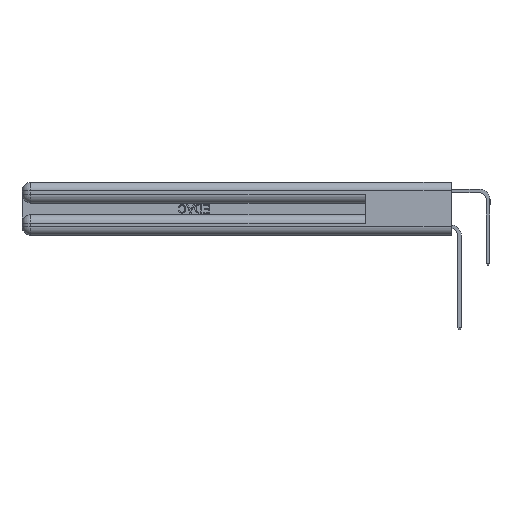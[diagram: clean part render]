
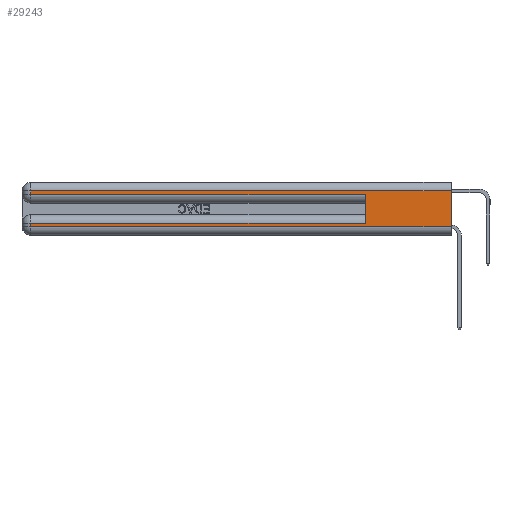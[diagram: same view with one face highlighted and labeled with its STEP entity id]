
A CAD part, left-side view. The second image highlights one B-rep face of the part: STEP entity #29243.
In plain terms, the highlighted planar face has unit normal (-1, 0, 0).
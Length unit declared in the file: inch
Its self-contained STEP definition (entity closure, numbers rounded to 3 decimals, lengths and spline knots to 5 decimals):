
#84 = LINE ( 'NONE', #25283, #3371 ) ;
#491 = LINE ( 'NONE', #1988, #9873 ) ;
#773 = EDGE_CURVE ( 'NONE', #15879, #17200, #33847, .T. ) ;
#850 = CARTESIAN_POINT ( 'NONE',  ( 0., 2.94, 0.37 ) ) ;
#945 = EDGE_LOOP ( 'NONE', ( #5033, #32286, #2455, #17928, #13160, #16162, #26212, #3657 ) ) ;
#1550 = CARTESIAN_POINT ( 'NONE',  ( 0., 2.94, 0.085 ) ) ;
#1559 = DIRECTION ( 'NONE',  ( 1., 0., 0. ) ) ;
#1988 = CARTESIAN_POINT ( 'NONE',  ( 0., 0., 0.085 ) ) ;
#2306 = CARTESIAN_POINT ( 'NONE',  ( 0., 2.94, 0.285 ) ) ;
#2379 = CARTESIAN_POINT ( 'NONE',  ( 0., 0.6, 0.085 ) ) ;
#2455 = ORIENTED_EDGE ( 'NONE', *, *, #14987, .T. ) ;
#3231 = LINE ( 'NONE', #850, #30244 ) ;
#3371 = VECTOR ( 'NONE', #14775, 39.37008 ) ;
#3577 = EDGE_CURVE ( 'NONE', #5012, #21733, #84, .T. ) ;
#3657 = ORIENTED_EDGE ( 'NONE', *, *, #11241, .T. ) ;
#4285 = CARTESIAN_POINT ( 'NONE',  ( 0., 0., 0.37 ) ) ;
#4335 = LINE ( 'NONE', #8128, #26035 ) ;
#4621 = VECTOR ( 'NONE', #21532, 39.37008 ) ;
#4627 = DIRECTION ( 'NONE',  ( 0., 0., -1. ) ) ;
#5012 = VERTEX_POINT ( 'NONE', #2306 ) ;
#5033 = ORIENTED_EDGE ( 'NONE', *, *, #9522, .F. ) ;
#5360 = VERTEX_POINT ( 'NONE', #2379 ) ;
#5896 = CARTESIAN_POINT ( 'NONE',  ( 0., 0., 0.31 ) ) ;
#7023 = PLANE ( 'NONE',  #14178 ) ;
#8128 = CARTESIAN_POINT ( 'NONE',  ( 0., 2.94, 0.37 ) ) ;
#9522 = EDGE_CURVE ( 'NONE', #15879, #20077, #25601, .T. ) ;
#9873 = VECTOR ( 'NONE', #12734, 39.37008 ) ;
#10524 = CARTESIAN_POINT ( 'NONE',  ( 0., 2.94, 0.06 ) ) ;
#10734 = DIRECTION ( 'NONE',  ( 0., 0., -1. ) ) ;
#11241 = EDGE_CURVE ( 'NONE', #26531, #20077, #11569, .T. ) ;
#11569 = LINE ( 'NONE', #19173, #4621 ) ;
#11875 = CARTESIAN_POINT ( 'NONE',  ( 0., 0., 0.31 ) ) ;
#12227 = FACE_OUTER_BOUND ( 'NONE', #945, .T. ) ;
#12734 = DIRECTION ( 'NONE',  ( 0., 1., 0. ) ) ;
#13160 = ORIENTED_EDGE ( 'NONE', *, *, #19964, .F. ) ;
#14178 = AXIS2_PLACEMENT_3D ( 'NONE', #4285, #1559, #27536 ) ;
#14775 = DIRECTION ( 'NONE',  ( 0., -1., 0. ) ) ;
#14987 = EDGE_CURVE ( 'NONE', #17200, #5012, #3231, .T. ) ;
#15879 = VERTEX_POINT ( 'NONE', #11875 ) ;
#16162 = ORIENTED_EDGE ( 'NONE', *, *, #20871, .T. ) ;
#16174 = DIRECTION ( 'NONE',  ( 0., 0., -1. ) ) ;
#16329 = CARTESIAN_POINT ( 'NONE',  ( 0., 2.94, 0.31 ) ) ;
#16333 = CARTESIAN_POINT ( 'NONE',  ( 0., 0.6, 0.145 ) ) ;
#16502 = EDGE_CURVE ( 'NONE', #26300, #26531, #4335, .T. ) ;
#17200 = VERTEX_POINT ( 'NONE', #16329 ) ;
#17928 = ORIENTED_EDGE ( 'NONE', *, *, #3577, .T. ) ;
#19173 = CARTESIAN_POINT ( 'NONE',  ( 0., 0., 0.06 ) ) ;
#19660 = CARTESIAN_POINT ( 'NONE',  ( 0., 0., 0.06 ) ) ;
#19964 = EDGE_CURVE ( 'NONE', #5360, #21733, #31975, .T. ) ;
#20077 = VERTEX_POINT ( 'NONE', #19660 ) ;
#20871 = EDGE_CURVE ( 'NONE', #5360, #26300, #491, .T. ) ;
#21076 = VECTOR ( 'NONE', #4627, 39.37008 ) ;
#21532 = DIRECTION ( 'NONE',  ( 0., -1., 0. ) ) ;
#21733 = VERTEX_POINT ( 'NONE', #29398 ) ;
#25283 = CARTESIAN_POINT ( 'NONE',  ( 0., 0., 0.285 ) ) ;
#25601 = LINE ( 'NONE', #27979, #21076 ) ;
#26035 = VECTOR ( 'NONE', #10734, 39.37008 ) ;
#26212 = ORIENTED_EDGE ( 'NONE', *, *, #16502, .T. ) ;
#26300 = VERTEX_POINT ( 'NONE', #1550 ) ;
#26531 = VERTEX_POINT ( 'NONE', #10524 ) ;
#27536 = DIRECTION ( 'NONE',  ( 0., 0., -1. ) ) ;
#27979 = CARTESIAN_POINT ( 'NONE',  ( 0., 0., 0.37 ) ) ;
#28040 = VECTOR ( 'NONE', #29038, 39.37008 ) ;
#28291 = VECTOR ( 'NONE', #29499, 39.37008 ) ;
#29038 = DIRECTION ( 'NONE',  ( 0., 1., 0. ) ) ;
#29243 = ADVANCED_FACE ( 'NONE', ( #12227 ), #7023, .F. ) ;
#29398 = CARTESIAN_POINT ( 'NONE',  ( 0., 0.6, 0.285 ) ) ;
#29499 = DIRECTION ( 'NONE',  ( 0., 0., 1. ) ) ;
#30244 = VECTOR ( 'NONE', #16174, 39.37008 ) ;
#31975 = LINE ( 'NONE', #16333, #28291 ) ;
#32286 = ORIENTED_EDGE ( 'NONE', *, *, #773, .T. ) ;
#33847 = LINE ( 'NONE', #5896, #28040 ) ;
